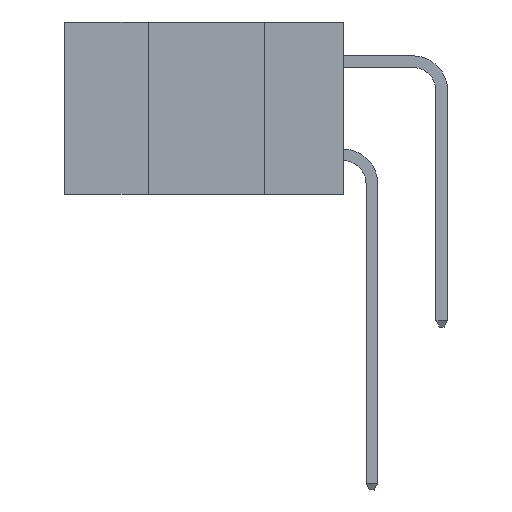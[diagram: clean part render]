
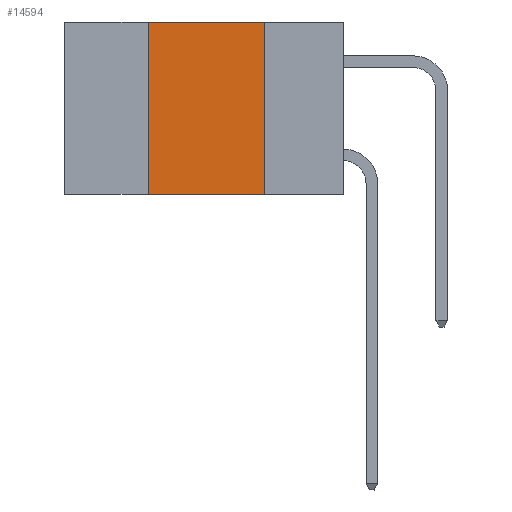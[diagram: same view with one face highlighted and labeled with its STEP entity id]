
A CAD part, left-side view. The second image highlights one B-rep face of the part: STEP entity #14594.
In plain terms, the highlighted planar face has unit normal (-1, 0, 0).
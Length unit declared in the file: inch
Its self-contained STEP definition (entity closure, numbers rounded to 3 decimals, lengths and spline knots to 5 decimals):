
#647 = VERTEX_POINT ( 'NONE', #24142 ) ;
#1150 = DIRECTION ( 'NONE',  ( 0., 0., -1. ) ) ;
#1826 = ORIENTED_EDGE ( 'NONE', *, *, #16064, .F. ) ;
#4143 = EDGE_CURVE ( 'NONE', #647, #21608, #29078, .T. ) ;
#4362 = AXIS2_PLACEMENT_3D ( 'NONE', #32892, #7496, #17492 ) ;
#4453 = CARTESIAN_POINT ( 'NONE',  ( 0., 0.42, 0. ) ) ;
#5068 = VECTOR ( 'NONE', #23913, 39.37008 ) ;
#7175 = PLANE ( 'NONE',  #4362 ) ;
#7496 = DIRECTION ( 'NONE',  ( 1., 0., 0. ) ) ;
#8790 = CARTESIAN_POINT ( 'NONE',  ( 0., 0.17, -0.37 ) ) ;
#11586 = CARTESIAN_POINT ( 'NONE',  ( 0., 0.17, 0. ) ) ;
#13929 = CARTESIAN_POINT ( 'NONE',  ( 0., 0.17, 0. ) ) ;
#13960 = EDGE_CURVE ( 'NONE', #31236, #21608, #14037, .T. ) ;
#14037 = LINE ( 'NONE', #13929, #23292 ) ;
#14594 = ADVANCED_FACE ( 'NONE', ( #20459 ), #7175, .F. ) ;
#16064 = EDGE_CURVE ( 'NONE', #27127, #31236, #18704, .T. ) ;
#16187 = ORIENTED_EDGE ( 'NONE', *, *, #4143, .T. ) ;
#17492 = DIRECTION ( 'NONE',  ( 0., 0., -1. ) ) ;
#18704 = LINE ( 'NONE', #26379, #5068 ) ;
#19099 = CARTESIAN_POINT ( 'NONE',  ( 0., 0.6, -0.37 ) ) ;
#19530 = ORIENTED_EDGE ( 'NONE', *, *, #13960, .F. ) ;
#20459 = FACE_OUTER_BOUND ( 'NONE', #25366, .T. ) ;
#21234 = VECTOR ( 'NONE', #30302, 39.37008 ) ;
#21608 = VERTEX_POINT ( 'NONE', #8790 ) ;
#22730 = ORIENTED_EDGE ( 'NONE', *, *, #28644, .F. ) ;
#23292 = VECTOR ( 'NONE', #1150, 39.37008 ) ;
#23913 = DIRECTION ( 'NONE',  ( 0., -1., 0. ) ) ;
#24142 = CARTESIAN_POINT ( 'NONE',  ( 0., 0.42, -0.37 ) ) ;
#25236 = CARTESIAN_POINT ( 'NONE',  ( 0., 0.42, 0. ) ) ;
#25366 = EDGE_LOOP ( 'NONE', ( #19530, #1826, #22730, #16187 ) ) ;
#26379 = CARTESIAN_POINT ( 'NONE',  ( 0., 0.6, 0. ) ) ;
#27127 = VERTEX_POINT ( 'NONE', #4453 ) ;
#28644 = EDGE_CURVE ( 'NONE', #647, #27127, #31279, .T. ) ;
#29078 = LINE ( 'NONE', #19099, #31842 ) ;
#30302 = DIRECTION ( 'NONE',  ( 0., 0., 1. ) ) ;
#31236 = VERTEX_POINT ( 'NONE', #11586 ) ;
#31279 = LINE ( 'NONE', #25236, #21234 ) ;
#31842 = VECTOR ( 'NONE', #32016, 39.37008 ) ;
#32016 = DIRECTION ( 'NONE',  ( 0., -1., 0. ) ) ;
#32892 = CARTESIAN_POINT ( 'NONE',  ( 0., 0.6, 0. ) ) ;
